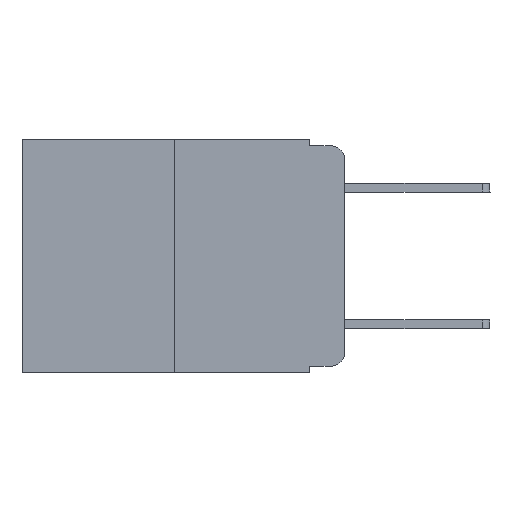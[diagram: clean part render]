
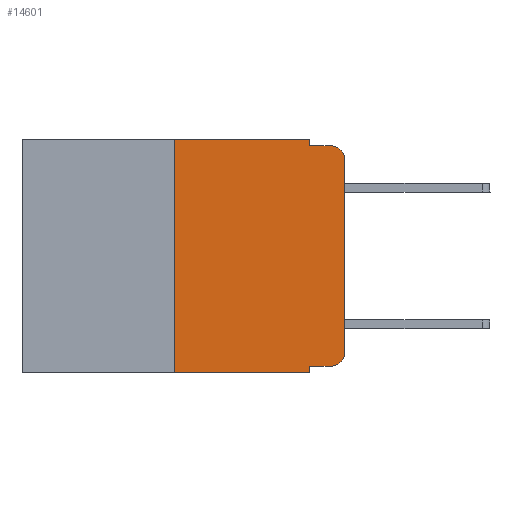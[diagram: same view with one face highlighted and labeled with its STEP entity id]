
A CAD part, left-side view. The second image highlights one B-rep face of the part: STEP entity #14601.
In plain terms, the highlighted planar face has unit normal (-1, 0, 0).
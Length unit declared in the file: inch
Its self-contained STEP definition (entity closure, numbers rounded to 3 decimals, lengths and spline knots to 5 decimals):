
#546 = EDGE_LOOP ( 'NONE', ( #13062, #8629, #13787, #23710, #19442, #23379, #12785, #15955, #22649, #23566 ) ) ;
#632 = VERTEX_POINT ( 'NONE', #23433 ) ;
#699 = VECTOR ( 'NONE', #13551, 39.37008 ) ;
#1292 = LINE ( 'NONE', #23934, #18348 ) ;
#1297 = CARTESIAN_POINT ( 'NONE',  ( 0., 0.25, 0. ) ) ;
#1505 = EDGE_CURVE ( 'NONE', #16586, #24311, #21167, .T. ) ;
#1747 = VERTEX_POINT ( 'NONE', #19920 ) ;
#2168 = LINE ( 'NONE', #19277, #8836 ) ;
#2220 = CARTESIAN_POINT ( 'NONE',  ( 0., 0.051, 0. ) ) ;
#2460 = FACE_OUTER_BOUND ( 'NONE', #546, .T. ) ;
#2772 = VERTEX_POINT ( 'NONE', #13305 ) ;
#2827 = DIRECTION ( 'NONE',  ( -1., 0., 0. ) ) ;
#2840 = DIRECTION ( 'NONE',  ( 0., -1., 0. ) ) ;
#3732 = VECTOR ( 'NONE', #13287, 39.37008 ) ;
#4313 = DIRECTION ( 'NONE',  ( 0., 0., -1. ) ) ;
#5890 = VECTOR ( 'NONE', #2840, 39.37008 ) ;
#6020 = EDGE_CURVE ( 'NONE', #9793, #2772, #15406, .T. ) ;
#6142 = CARTESIAN_POINT ( 'NONE',  ( 0., 0.02, -0.03 ) ) ;
#6156 = PLANE ( 'NONE',  #19792 ) ;
#7219 = DIRECTION ( 'NONE',  ( 0., 0., -1. ) ) ;
#8089 = CARTESIAN_POINT ( 'NONE',  ( 0., 0.473, 0. ) ) ;
#8216 = DIRECTION ( 'NONE',  ( 0., -1., 0. ) ) ;
#8322 = AXIS2_PLACEMENT_3D ( 'NONE', #24067, #8929, #7219 ) ;
#8629 = ORIENTED_EDGE ( 'NONE', *, *, #1505, .T. ) ;
#8717 = CIRCLE ( 'NONE', #8322, 0.02 ) ;
#8836 = VECTOR ( 'NONE', #17428, 39.37008 ) ;
#8929 = DIRECTION ( 'NONE',  ( -1., 0., 0. ) ) ;
#9418 = EDGE_CURVE ( 'NONE', #16531, #1747, #14053, .T. ) ;
#9746 = DIRECTION ( 'NONE',  ( 0., 0., -1. ) ) ;
#9793 = VERTEX_POINT ( 'NONE', #11675 ) ;
#10529 = EDGE_CURVE ( 'NONE', #9793, #23821, #24052, .T. ) ;
#10896 = DIRECTION ( 'NONE',  ( 0., 0., -1. ) ) ;
#11675 = CARTESIAN_POINT ( 'NONE',  ( 0., 0.25, -0.343 ) ) ;
#12785 = ORIENTED_EDGE ( 'NONE', *, *, #6020, .T. ) ;
#12958 = AXIS2_PLACEMENT_3D ( 'NONE', #6142, #2827, #4313 ) ;
#13062 = ORIENTED_EDGE ( 'NONE', *, *, #19429, .T. ) ;
#13287 = DIRECTION ( 'NONE',  ( 0., -1., 0. ) ) ;
#13305 = CARTESIAN_POINT ( 'NONE',  ( 0., 0.051, -0.343 ) ) ;
#13435 = LINE ( 'NONE', #2220, #17920 ) ;
#13439 = EDGE_CURVE ( 'NONE', #1747, #15677, #8717, .T. ) ;
#13551 = DIRECTION ( 'NONE',  ( 0., -1., 0. ) ) ;
#13787 = ORIENTED_EDGE ( 'NONE', *, *, #23175, .F. ) ;
#14053 = LINE ( 'NONE', #21773, #5890 ) ;
#14601 = ADVANCED_FACE ( 'NONE', ( #2460 ), #6156, .F. ) ;
#14895 = CARTESIAN_POINT ( 'NONE',  ( 0., 0.02, -0.01 ) ) ;
#14964 = VECTOR ( 'NONE', #19880, 39.37008 ) ;
#15386 = LINE ( 'NONE', #21022, #19922 ) ;
#15406 = LINE ( 'NONE', #22886, #699 ) ;
#15532 = CARTESIAN_POINT ( 'NONE',  ( 0., 0.473, 0. ) ) ;
#15677 = VERTEX_POINT ( 'NONE', #20450 ) ;
#15714 = CARTESIAN_POINT ( 'NONE',  ( 0., 0.051, -0.333 ) ) ;
#15955 = ORIENTED_EDGE ( 'NONE', *, *, #22557, .F. ) ;
#16023 = DIRECTION ( 'NONE',  ( 0., 0., -1. ) ) ;
#16531 = VERTEX_POINT ( 'NONE', #15714 ) ;
#16586 = VERTEX_POINT ( 'NONE', #20774 ) ;
#17428 = DIRECTION ( 'NONE',  ( 0., 0., 1. ) ) ;
#17549 = CARTESIAN_POINT ( 'NONE',  ( 0., 0.051, -0.01 ) ) ;
#17680 = CARTESIAN_POINT ( 'NONE',  ( 0., 0.25, 0. ) ) ;
#17920 = VECTOR ( 'NONE', #9746, 39.37008 ) ;
#18348 = VECTOR ( 'NONE', #10896, 39.37008 ) ;
#19002 = EDGE_CURVE ( 'NONE', #23821, #632, #22989, .T. ) ;
#19277 = CARTESIAN_POINT ( 'NONE',  ( 0., 0., 0. ) ) ;
#19429 = EDGE_CURVE ( 'NONE', #15677, #16586, #2168, .T. ) ;
#19442 = ORIENTED_EDGE ( 'NONE', *, *, #19002, .F. ) ;
#19566 = VERTEX_POINT ( 'NONE', #17549 ) ;
#19792 = AXIS2_PLACEMENT_3D ( 'NONE', #15532, #23392, #16023 ) ;
#19880 = DIRECTION ( 'NONE',  ( 0., 0., 1. ) ) ;
#19920 = CARTESIAN_POINT ( 'NONE',  ( 0., 0.02, -0.333 ) ) ;
#19922 = VECTOR ( 'NONE', #8216, 39.37008 ) ;
#20450 = CARTESIAN_POINT ( 'NONE',  ( 0., 0., -0.313 ) ) ;
#20774 = CARTESIAN_POINT ( 'NONE',  ( 0., 0., -0.03 ) ) ;
#21022 = CARTESIAN_POINT ( 'NONE',  ( 0., 0.051, -0.01 ) ) ;
#21167 = CIRCLE ( 'NONE', #12958, 0.02 ) ;
#21498 = EDGE_CURVE ( 'NONE', #632, #19566, #13435, .T. ) ;
#21773 = CARTESIAN_POINT ( 'NONE',  ( 0., 0.051, -0.333 ) ) ;
#22557 = EDGE_CURVE ( 'NONE', #16531, #2772, #1292, .T. ) ;
#22649 = ORIENTED_EDGE ( 'NONE', *, *, #9418, .T. ) ;
#22886 = CARTESIAN_POINT ( 'NONE',  ( 0., 0.473, -0.343 ) ) ;
#22989 = LINE ( 'NONE', #8089, #3732 ) ;
#23175 = EDGE_CURVE ( 'NONE', #19566, #24311, #15386, .T. ) ;
#23379 = ORIENTED_EDGE ( 'NONE', *, *, #10529, .F. ) ;
#23392 = DIRECTION ( 'NONE',  ( 1., 0., 0. ) ) ;
#23433 = CARTESIAN_POINT ( 'NONE',  ( 0., 0.051, 0. ) ) ;
#23566 = ORIENTED_EDGE ( 'NONE', *, *, #13439, .T. ) ;
#23710 = ORIENTED_EDGE ( 'NONE', *, *, #21498, .F. ) ;
#23821 = VERTEX_POINT ( 'NONE', #17680 ) ;
#23934 = CARTESIAN_POINT ( 'NONE',  ( 0., 0.051, 0. ) ) ;
#24052 = LINE ( 'NONE', #1297, #14964 ) ;
#24067 = CARTESIAN_POINT ( 'NONE',  ( 0., 0.02, -0.313 ) ) ;
#24311 = VERTEX_POINT ( 'NONE', #14895 ) ;
